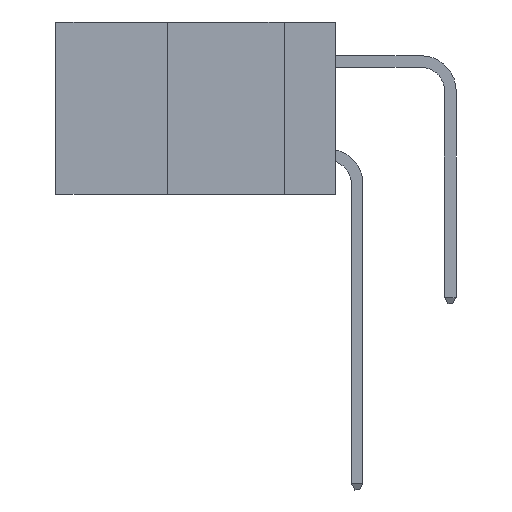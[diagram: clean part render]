
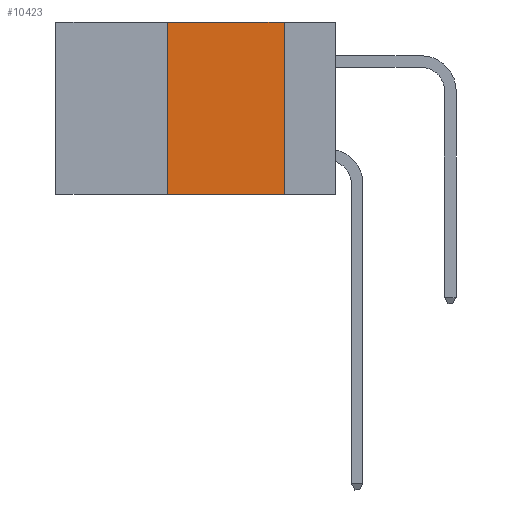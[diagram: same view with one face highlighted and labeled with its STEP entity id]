
A CAD part, left-side view. The second image highlights one B-rep face of the part: STEP entity #10423.
In plain terms, the highlighted planar face has unit normal (-1, 0, 0).
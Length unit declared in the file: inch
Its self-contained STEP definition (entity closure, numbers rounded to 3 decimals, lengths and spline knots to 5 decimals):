
#467 = DIRECTION ( 'NONE',  ( 0., -1., 0. ) ) ;
#1768 = DIRECTION ( 'NONE',  ( 0., -1., 0. ) ) ;
#1865 = CARTESIAN_POINT ( 'NONE',  ( 0., 0.6, 0. ) ) ;
#4049 = LINE ( 'NONE', #7608, #5767 ) ;
#4182 = DIRECTION ( 'NONE',  ( 0., 0., 1. ) ) ;
#4198 = ORIENTED_EDGE ( 'NONE', *, *, #10261, .F. ) ;
#4209 = CARTESIAN_POINT ( 'NONE',  ( 0., 0.6, 0. ) ) ;
#4587 = FACE_OUTER_BOUND ( 'NONE', #6725, .T. ) ;
#5322 = CARTESIAN_POINT ( 'NONE',  ( 0., 0.36, 0. ) ) ;
#5708 = VECTOR ( 'NONE', #1768, 39.37008 ) ;
#5767 = VECTOR ( 'NONE', #7446, 39.37008 ) ;
#6271 = VECTOR ( 'NONE', #4182, 39.37008 ) ;
#6725 = EDGE_LOOP ( 'NONE', ( #12866, #8236, #4198, #8068 ) ) ;
#6809 = LINE ( 'NONE', #4209, #8452 ) ;
#7446 = DIRECTION ( 'NONE',  ( 0., 0., -1. ) ) ;
#7591 = CARTESIAN_POINT ( 'NONE',  ( 0., 0.36, 0. ) ) ;
#7608 = CARTESIAN_POINT ( 'NONE',  ( 0., 0.11, 0. ) ) ;
#8068 = ORIENTED_EDGE ( 'NONE', *, *, #13734, .T. ) ;
#8236 = ORIENTED_EDGE ( 'NONE', *, *, #11701, .F. ) ;
#8452 = VECTOR ( 'NONE', #467, 39.37008 ) ;
#9232 = VERTEX_POINT ( 'NONE', #14330 ) ;
#9466 = CARTESIAN_POINT ( 'NONE',  ( 0., 0.11, 0. ) ) ;
#10035 = VERTEX_POINT ( 'NONE', #9466 ) ;
#10261 = EDGE_CURVE ( 'NONE', #10695, #15665, #13624, .T. ) ;
#10423 = ADVANCED_FACE ( 'NONE', ( #4587 ), #10525, .F. ) ;
#10525 = PLANE ( 'NONE',  #12224 ) ;
#10695 = VERTEX_POINT ( 'NONE', #12347 ) ;
#11642 = DIRECTION ( 'NONE',  ( 1., 0., 0. ) ) ;
#11701 = EDGE_CURVE ( 'NONE', #15665, #10035, #6809, .T. ) ;
#12224 = AXIS2_PLACEMENT_3D ( 'NONE', #1865, #11642, #14250 ) ;
#12347 = CARTESIAN_POINT ( 'NONE',  ( 0., 0.36, -0.37 ) ) ;
#12654 = LINE ( 'NONE', #15249, #5708 ) ;
#12866 = ORIENTED_EDGE ( 'NONE', *, *, #15598, .F. ) ;
#13624 = LINE ( 'NONE', #7591, #6271 ) ;
#13734 = EDGE_CURVE ( 'NONE', #10695, #9232, #12654, .T. ) ;
#14250 = DIRECTION ( 'NONE',  ( 0., 0., -1. ) ) ;
#14330 = CARTESIAN_POINT ( 'NONE',  ( 0., 0.11, -0.37 ) ) ;
#15249 = CARTESIAN_POINT ( 'NONE',  ( 0., 0.6, -0.37 ) ) ;
#15598 = EDGE_CURVE ( 'NONE', #10035, #9232, #4049, .T. ) ;
#15665 = VERTEX_POINT ( 'NONE', #5322 ) ;
